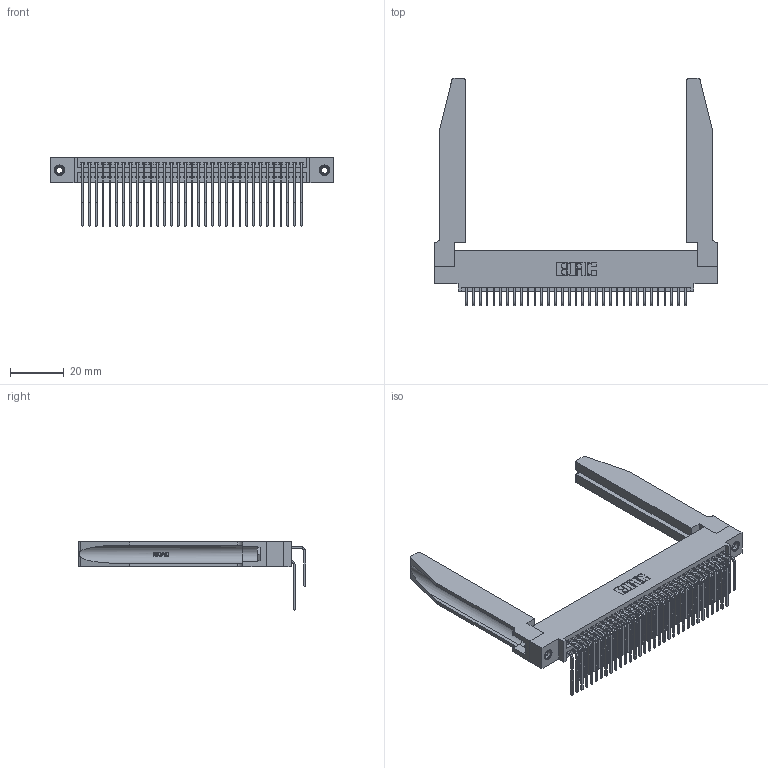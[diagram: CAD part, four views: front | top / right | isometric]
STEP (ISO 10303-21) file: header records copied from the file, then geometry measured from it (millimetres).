
FILE_DESCRIPTION (( 'STEP AP203' ), '1' );
FILE_NAME ('345-066-559-578.STEP', '2019-10-30T18:42:55', ( '' ), ( '' ), 'SwSTEP 2.0', 'SolidWorks 2016', '' );
FILE_SCHEMA (( 'CONFIG_CONTROL_DESIGN' ));
Length unit declared in the file: inch
Products named in the file (6): 345-250-001_345-250-001-102; 345-292-001_558 559 Tail - 1; 345-066-559-578; 345-220-078_345-220-078; 345 Part_0.110 Offset - 0.156 Dia-TH; 345-292-001_559 Tail - 2
Assembly tree (71 placements, depth 2):
  345-066-559-578
    345 Part_0.110 Offset - 0.156 Dia-TH
    345-292-001_558 559 Tail - 1  x33
    345-292-001_559 Tail - 2  x33
    345-250-001_345-250-001-102  x2
    345-220-078_345-220-078  x2
Bounding box: 105.05 x 84.32 x 25.53 mm (x, y, z)
Volume: 18199.4 mm3; surface area: 23963 mm2
Topology: 71 solids, 71 shells, 3796 faces, 11191 edges, 7362 vertices
Faces by surface type: plane 2536, cylinder 1208, bspline 36, cone 12, torus 4
Entity records: 33628 total; most frequent: CARTESIAN_POINT 6610, ORIENTED_EDGE 5390, DIRECTION 4805, EDGE_CURVE 2695, LINE 2297, VECTOR 2297, VERTEX_POINT 1788, AXIS2_PLACEMENT_3D 1254
